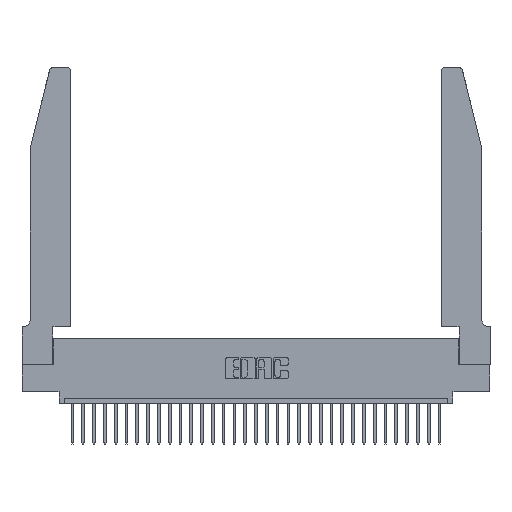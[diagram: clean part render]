
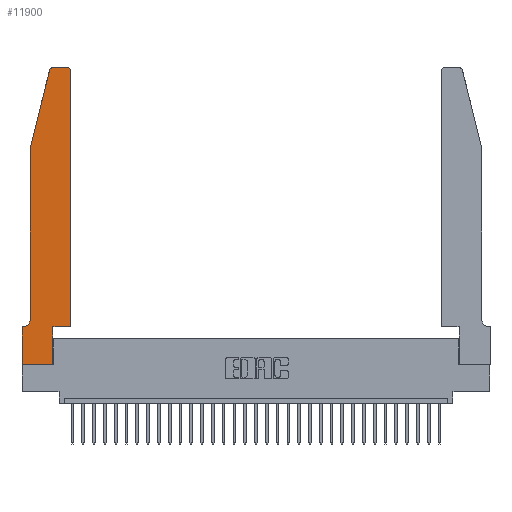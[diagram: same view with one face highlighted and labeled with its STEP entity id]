
A CAD part, top view. The second image highlights one B-rep face of the part: STEP entity #11900.
In plain terms, the highlighted planar face has unit normal (0, 0, 1).
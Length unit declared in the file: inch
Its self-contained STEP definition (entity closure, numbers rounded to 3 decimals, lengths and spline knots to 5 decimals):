
#677 = DIRECTION ( 'NONE',  ( -0.239, -0.971, 0. ) ) ;
#1382 = EDGE_CURVE ( 'NONE', #13301, #27997, #12606, .T. ) ;
#1642 = CARTESIAN_POINT ( 'NONE',  ( 0.0755, 2., 0.37 ) ) ;
#2130 = AXIS2_PLACEMENT_3D ( 'NONE', #8426, #3025, #14364 ) ;
#2366 = ORIENTED_EDGE ( 'NONE', *, *, #13448, .T. ) ;
#2708 = EDGE_CURVE ( 'NONE', #27997, #6894, #10663, .T. ) ;
#3025 = DIRECTION ( 'NONE',  ( 0., 0., 1. ) ) ;
#3155 = CARTESIAN_POINT ( 'NONE',  ( 0., 0., 0.37 ) ) ;
#3593 = VECTOR ( 'NONE', #677, 39.37008 ) ;
#3674 = LINE ( 'NONE', #17066, #5223 ) ;
#4742 = CARTESIAN_POINT ( 'NONE',  ( 0.4205, 2.75, 0.37 ) ) ;
#4852 = DIRECTION ( 'NONE',  ( -1., 0., 0. ) ) ;
#4971 = VERTEX_POINT ( 'NONE', #28126 ) ;
#4972 = EDGE_CURVE ( 'NONE', #13218, #13301, #12353, .T. ) ;
#5223 = VECTOR ( 'NONE', #29138, 39.37008 ) ;
#5775 = VECTOR ( 'NONE', #10792, 39.37008 ) ;
#5889 = CARTESIAN_POINT ( 'NONE',  ( 0.4505, 0.35, 0.37 ) ) ;
#5979 = EDGE_CURVE ( 'NONE', #12970, #11122, #19278, .T. ) ;
#6028 = DIRECTION ( 'NONE',  ( -1., 0., 0. ) ) ;
#6598 = CARTESIAN_POINT ( 'NONE',  ( 0.25487, 2.72718, 0.37 ) ) ;
#6637 = LINE ( 'NONE', #12972, #9752 ) ;
#6656 = EDGE_CURVE ( 'NONE', #8930, #27471, #31293, .T. ) ;
#6894 = VERTEX_POINT ( 'NONE', #20052 ) ;
#7064 = LINE ( 'NONE', #1642, #21023 ) ;
#7366 = LINE ( 'NONE', #25423, #24427 ) ;
#7384 = AXIS2_PLACEMENT_3D ( 'NONE', #9866, #27092, #4852 ) ;
#7587 = EDGE_CURVE ( 'NONE', #6894, #4971, #23028, .T. ) ;
#7627 = DIRECTION ( 'NONE',  ( 1., 0., 0. ) ) ;
#7866 = ORIENTED_EDGE ( 'NONE', *, *, #11472, .T. ) ;
#8346 = VERTEX_POINT ( 'NONE', #20239 ) ;
#8426 = CARTESIAN_POINT ( 'NONE',  ( 0.284, 2.72, 0.37 ) ) ;
#8500 = CARTESIAN_POINT ( 'NONE',  ( 0., 0., 0.37 ) ) ;
#8674 = EDGE_CURVE ( 'NONE', #22801, #8346, #7064, .T. ) ;
#8930 = VERTEX_POINT ( 'NONE', #28130 ) ;
#9752 = VECTOR ( 'NONE', #6028, 39.37008 ) ;
#9866 = CARTESIAN_POINT ( 'NONE',  ( 0.0055, 0.42, 0.37 ) ) ;
#10201 = LINE ( 'NONE', #30425, #3593 ) ;
#10663 = LINE ( 'NONE', #25621, #15672 ) ;
#10712 = DIRECTION ( 'NONE',  ( 1., 0., 0. ) ) ;
#10792 = DIRECTION ( 'NONE',  ( 0., -1., 0. ) ) ;
#11122 = VERTEX_POINT ( 'NONE', #6598 ) ;
#11472 = EDGE_CURVE ( 'NONE', #4971, #8930, #3674, .T. ) ;
#11900 = ADVANCED_FACE ( 'NONE', ( #25727 ), #12821, .T. ) ;
#12353 = LINE ( 'NONE', #8500, #5775 ) ;
#12606 = LINE ( 'NONE', #3155, #29313 ) ;
#12821 = PLANE ( 'NONE',  #20638 ) ;
#12970 = VERTEX_POINT ( 'NONE', #20411 ) ;
#12972 = CARTESIAN_POINT ( 'NONE',  ( 0.2605, 2.75, 0.37 ) ) ;
#13218 = VERTEX_POINT ( 'NONE', #24672 ) ;
#13301 = VERTEX_POINT ( 'NONE', #17645 ) ;
#13354 = ORIENTED_EDGE ( 'NONE', *, *, #14110, .T. ) ;
#13448 = EDGE_CURVE ( 'NONE', #27471, #12970, #6637, .T. ) ;
#13604 = CARTESIAN_POINT ( 'NONE',  ( 0.0755, 2., 0.37 ) ) ;
#14110 = EDGE_CURVE ( 'NONE', #8346, #30898, #30671, .T. ) ;
#14364 = DIRECTION ( 'NONE',  ( 1., 0., 0. ) ) ;
#15176 = DIRECTION ( 'NONE',  ( 0., 0., 1. ) ) ;
#15639 = AXIS2_PLACEMENT_3D ( 'NONE', #24319, #15176, #10712 ) ;
#15672 = VECTOR ( 'NONE', #30525, 39.37008 ) ;
#17066 = CARTESIAN_POINT ( 'NONE',  ( 0.4505, 0.35, 0.37 ) ) ;
#17645 = CARTESIAN_POINT ( 'NONE',  ( 0., 0., 0.37 ) ) ;
#18728 = CARTESIAN_POINT ( 'NONE',  ( 0.2865, 0., 0.37 ) ) ;
#18811 = DIRECTION ( 'NONE',  ( -1., 0., 0. ) ) ;
#18996 = DIRECTION ( 'NONE',  ( 0., -1., 0. ) ) ;
#19278 = CIRCLE ( 'NONE', #2130, 0.03 ) ;
#19409 = ORIENTED_EDGE ( 'NONE', *, *, #25083, .T. ) ;
#19787 = CARTESIAN_POINT ( 'NONE',  ( 0.0055, 0.35, 0.37 ) ) ;
#20052 = CARTESIAN_POINT ( 'NONE',  ( 0.2865, 0.35, 0.37 ) ) ;
#20202 = CARTESIAN_POINT ( 'NONE',  ( 0., 0.35, 0.37 ) ) ;
#20239 = CARTESIAN_POINT ( 'NONE',  ( 0.0755, 0.42, 0.37 ) ) ;
#20250 = ORIENTED_EDGE ( 'NONE', *, *, #1382, .T. ) ;
#20411 = CARTESIAN_POINT ( 'NONE',  ( 0.284, 2.75, 0.37 ) ) ;
#20492 = DIRECTION ( 'NONE',  ( 1., 0., 0. ) ) ;
#20638 = AXIS2_PLACEMENT_3D ( 'NONE', #20202, #22803, #7627 ) ;
#21023 = VECTOR ( 'NONE', #18996, 39.37008 ) ;
#21262 = ORIENTED_EDGE ( 'NONE', *, *, #26558, .T. ) ;
#21877 = ORIENTED_EDGE ( 'NONE', *, *, #8674, .T. ) ;
#22799 = DIRECTION ( 'NONE',  ( 1., 0., 0. ) ) ;
#22801 = VERTEX_POINT ( 'NONE', #13604 ) ;
#22803 = DIRECTION ( 'NONE',  ( 0., 0., 1. ) ) ;
#23028 = LINE ( 'NONE', #5889, #30442 ) ;
#24319 = CARTESIAN_POINT ( 'NONE',  ( 0.4205, 2.72, 0.37 ) ) ;
#24427 = VECTOR ( 'NONE', #18811, 39.37008 ) ;
#24672 = CARTESIAN_POINT ( 'NONE',  ( 0., 0.35, 0.37 ) ) ;
#25083 = EDGE_CURVE ( 'NONE', #30898, #13218, #7366, .T. ) ;
#25423 = CARTESIAN_POINT ( 'NONE',  ( 0.0755, 0.35, 0.37 ) ) ;
#25621 = CARTESIAN_POINT ( 'NONE',  ( 0.2865, 0.35, 0.37 ) ) ;
#25727 = FACE_OUTER_BOUND ( 'NONE', #25958, .T. ) ;
#25958 = EDGE_LOOP ( 'NONE', ( #2366, #29849, #21262, #21877, #13354, #19409, #28793, #20250, #31054, #28040, #7866, #31886 ) ) ;
#26558 = EDGE_CURVE ( 'NONE', #11122, #22801, #10201, .T. ) ;
#27092 = DIRECTION ( 'NONE',  ( 0., 0., -1. ) ) ;
#27471 = VERTEX_POINT ( 'NONE', #4742 ) ;
#27997 = VERTEX_POINT ( 'NONE', #18728 ) ;
#28040 = ORIENTED_EDGE ( 'NONE', *, *, #7587, .T. ) ;
#28126 = CARTESIAN_POINT ( 'NONE',  ( 0.4505, 0.35, 0.37 ) ) ;
#28130 = CARTESIAN_POINT ( 'NONE',  ( 0.4505, 2.72, 0.37 ) ) ;
#28793 = ORIENTED_EDGE ( 'NONE', *, *, #4972, .T. ) ;
#29138 = DIRECTION ( 'NONE',  ( 0., 1., 0. ) ) ;
#29313 = VECTOR ( 'NONE', #20492, 39.37008 ) ;
#29849 = ORIENTED_EDGE ( 'NONE', *, *, #5979, .T. ) ;
#30425 = CARTESIAN_POINT ( 'NONE',  ( 0.0755, 2., 0.37 ) ) ;
#30442 = VECTOR ( 'NONE', #22799, 39.37008 ) ;
#30525 = DIRECTION ( 'NONE',  ( 0., 1., 0. ) ) ;
#30671 = CIRCLE ( 'NONE', #7384, 0.07 ) ;
#30898 = VERTEX_POINT ( 'NONE', #19787 ) ;
#31054 = ORIENTED_EDGE ( 'NONE', *, *, #2708, .T. ) ;
#31293 = CIRCLE ( 'NONE', #15639, 0.03 ) ;
#31886 = ORIENTED_EDGE ( 'NONE', *, *, #6656, .T. ) ;
